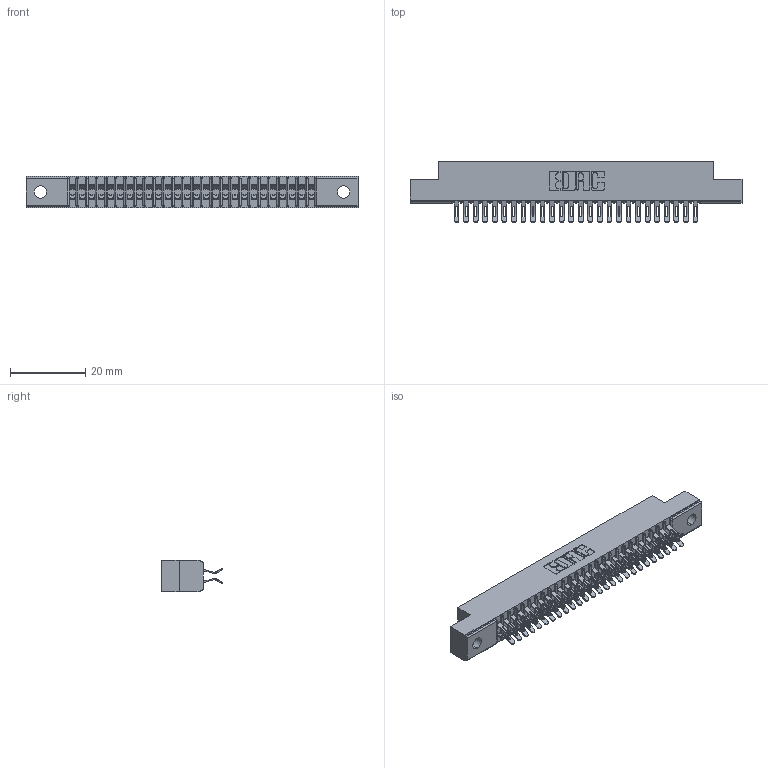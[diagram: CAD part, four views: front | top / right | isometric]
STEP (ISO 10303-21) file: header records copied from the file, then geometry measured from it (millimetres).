
FILE_DESCRIPTION (( 'STEP AP203' ), '1' );
FILE_NAME ('391-052-555-202.STEP', '2018-08-09T06:18:11', ( '' ), ( '' ), 'SwSTEP 2.0', 'SolidWorks 2016', '' );
FILE_SCHEMA (( 'CONFIG_CONTROL_DESIGN' ));
Length unit declared in the file: inch
Products named in the file (3): 391-052-555-202; 341 Part_.128 (3.25) Dia Mounting Holes; 341-292-001_341-292-155
Assembly tree (53 placements, depth 2):
  391-052-555-202
    341 Part_.128 (3.25) Dia Mounting Holes
    341-292-001_341-292-155  x52
Bounding box: 88.27 x 16.31 x 8.38 mm (x, y, z)
Volume: 5040.1 mm3; surface area: 10909.1 mm2
Topology: 53 solids, 53 shells, 4172 faces, 12458 edges, 8110 vertices
Faces by surface type: plane 2252, cylinder 1816, sphere 54, torus 50
Entity records: 34069 total; most frequent: CARTESIAN_POINT 5680, ORIENTED_EDGE 5632, DIRECTION 5514, EDGE_CURVE 2816, VECTOR 2242, LINE 2242, VERTEX_POINT 1786, AXIS2_PLACEMENT_3D 1636
